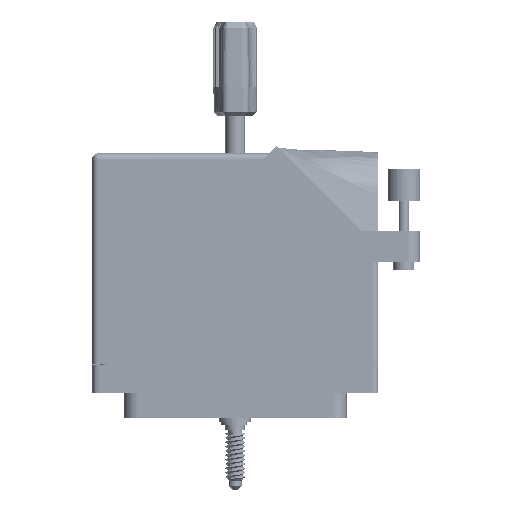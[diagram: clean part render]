
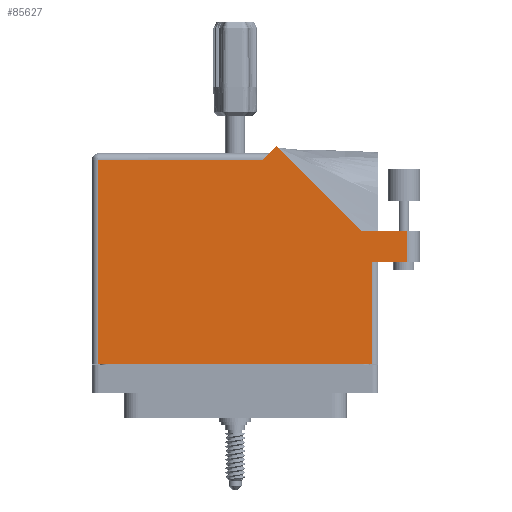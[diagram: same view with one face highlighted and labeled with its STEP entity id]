
A CAD part, front view. The second image highlights one B-rep face of the part: STEP entity #85627.
In plain terms, the highlighted face is planar.
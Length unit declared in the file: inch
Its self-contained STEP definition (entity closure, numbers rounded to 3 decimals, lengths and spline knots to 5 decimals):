
#1533 = VERTEX_POINT ( 'NONE', #86568 ) ;
#3711 = VERTEX_POINT ( 'NONE', #14160 ) ;
#5262 = DIRECTION ( 'NONE',  ( 1., 0., 0. ) ) ;
#7871 = VECTOR ( 'NONE', #48670, 39.37008 ) ;
#8618 = VECTOR ( 'NONE', #37845, 39.37008 ) ;
#8936 = DIRECTION ( 'NONE',  ( -1., 0., 0. ) ) ;
#9308 = CARTESIAN_POINT ( 'NONE',  ( 1.7775, 1.187, 0.765 ) ) ;
#9536 = CARTESIAN_POINT ( 'NONE',  ( 1.6525, 0.88, 0.765 ) ) ;
#9553 = LINE ( 'NONE', #60738, #47862 ) ;
#10353 = ORIENTED_EDGE ( 'NONE', *, *, #39076, .T. ) ;
#11159 = DIRECTION ( 'NONE',  ( 0., 1., 0. ) ) ;
#12064 = VERTEX_POINT ( 'NONE', #9536 ) ;
#12413 = VERTEX_POINT ( 'NONE', #81875 ) ;
#12888 = ORIENTED_EDGE ( 'NONE', *, *, #55813, .T. ) ;
#14160 = CARTESIAN_POINT ( 'NONE',  ( 0.39821, 2.00071, 0.765 ) ) ;
#15164 = VERTEX_POINT ( 'NONE', #15915 ) ;
#15915 = CARTESIAN_POINT ( 'NONE',  ( 1.21192, 1.187, 0.765 ) ) ;
#18569 = EDGE_CURVE ( 'NONE', #64578, #12064, #103659, .T. ) ;
#19129 = CARTESIAN_POINT ( 'NONE',  ( 1.21192, 1.187, 0.765 ) ) ;
#21753 = CARTESIAN_POINT ( 'NONE',  ( -1.3155, -0.1, 0.765 ) ) ;
#22735 = LINE ( 'NONE', #62790, #8618 ) ;
#22827 = VERTEX_POINT ( 'NONE', #45291 ) ;
#23236 = ORIENTED_EDGE ( 'NONE', *, *, #60912, .T. ) ;
#25490 = DIRECTION ( 'NONE',  ( -0.707, -0.707, 0. ) ) ;
#25678 = LINE ( 'NONE', #64691, #7871 ) ;
#25749 = ORIENTED_EDGE ( 'NONE', *, *, #65147, .T. ) ;
#27360 = CARTESIAN_POINT ( 'NONE',  ( -1.3155, 1.868, 0.765 ) ) ;
#29050 = VERTEX_POINT ( 'NONE', #27360 ) ;
#29961 = DIRECTION ( 'NONE',  ( 0., -1., 0. ) ) ;
#31330 = LINE ( 'NONE', #98326, #93917 ) ;
#32808 = ORIENTED_EDGE ( 'NONE', *, *, #70916, .T. ) ;
#34375 = VECTOR ( 'NONE', #29961, 39.37008 ) ;
#34515 = EDGE_CURVE ( 'NONE', #12064, #12413, #25678, .T. ) ;
#35203 = DIRECTION ( 'NONE',  ( -0.707, 0.707, 0. ) ) ;
#37845 = DIRECTION ( 'NONE',  ( -1., 0., 0. ) ) ;
#39076 = EDGE_CURVE ( 'NONE', #3711, #1533, #31330, .T. ) ;
#42021 = CARTESIAN_POINT ( 'NONE',  ( -1.3775, 1.93, 0.765 ) ) ;
#42851 = DIRECTION ( 'NONE',  ( 0., 0., -1. ) ) ;
#45291 = CARTESIAN_POINT ( 'NONE',  ( -1.3155, -0.1, 0.765 ) ) ;
#47862 = VECTOR ( 'NONE', #11159, 39.37008 ) ;
#48670 = DIRECTION ( 'NONE',  ( 0., 1., 0. ) ) ;
#49932 = VECTOR ( 'NONE', #5262, 39.37008 ) ;
#50260 = CARTESIAN_POINT ( 'NONE',  ( 1.3775, 0.88, 0.765 ) ) ;
#51410 = AXIS2_PLACEMENT_3D ( 'NONE', #42021, #42851, #99990 ) ;
#52316 = VERTEX_POINT ( 'NONE', #105827 ) ;
#53189 = LINE ( 'NONE', #19129, #94052 ) ;
#55813 = EDGE_CURVE ( 'NONE', #15164, #3711, #53189, .T. ) ;
#57748 = ORIENTED_EDGE ( 'NONE', *, *, #34515, .T. ) ;
#60051 = ORIENTED_EDGE ( 'NONE', *, *, #105525, .T. ) ;
#60738 = CARTESIAN_POINT ( 'NONE',  ( 1.3155, 0.88, 0.765 ) ) ;
#60912 = EDGE_CURVE ( 'NONE', #29050, #22827, #82968, .T. ) ;
#62097 = VECTOR ( 'NONE', #8936, 39.37008 ) ;
#62790 = CARTESIAN_POINT ( 'NONE',  ( -1.3775, 1.868, 0.765 ) ) ;
#63529 = CARTESIAN_POINT ( 'NONE',  ( 1.3155, 0.88, 0.765 ) ) ;
#63993 = ORIENTED_EDGE ( 'NONE', *, *, #18569, .T. ) ;
#64578 = VERTEX_POINT ( 'NONE', #63529 ) ;
#64691 = CARTESIAN_POINT ( 'NONE',  ( 1.6525, 1.187, 0.765 ) ) ;
#65147 = EDGE_CURVE ( 'NONE', #22827, #52316, #71584, .T. ) ;
#70916 = EDGE_CURVE ( 'NONE', #52316, #64578, #9553, .T. ) ;
#71584 = LINE ( 'NONE', #102746, #49932 ) ;
#79349 = FACE_OUTER_BOUND ( 'NONE', #92042, .T. ) ;
#81875 = CARTESIAN_POINT ( 'NONE',  ( 1.6525, 1.187, 0.765 ) ) ;
#82968 = LINE ( 'NONE', #21753, #34375 ) ;
#85627 = ADVANCED_FACE ( 'NONE', ( #79349 ), #91626, .F. ) ;
#86470 = ORIENTED_EDGE ( 'NONE', *, *, #104288, .T. ) ;
#86568 = CARTESIAN_POINT ( 'NONE',  ( 0.2655, 1.868, 0.765 ) ) ;
#90214 = DIRECTION ( 'NONE',  ( 1., 0., 0. ) ) ;
#91626 = PLANE ( 'NONE',  #51410 ) ;
#92042 = EDGE_LOOP ( 'NONE', ( #63993, #57748, #60051, #12888, #10353, #86470, #23236, #25749, #32808 ) ) ;
#93917 = VECTOR ( 'NONE', #25490, 39.37008 ) ;
#94052 = VECTOR ( 'NONE', #35203, 39.37008 ) ;
#98326 = CARTESIAN_POINT ( 'NONE',  ( 0.3275, 1.93, 0.765 ) ) ;
#99990 = DIRECTION ( 'NONE',  ( -1., 0., 0. ) ) ;
#101100 = VECTOR ( 'NONE', #90214, 39.37008 ) ;
#102746 = CARTESIAN_POINT ( 'NONE',  ( -1.3775, -0.1, 0.765 ) ) ;
#103659 = LINE ( 'NONE', #50260, #101100 ) ;
#104288 = EDGE_CURVE ( 'NONE', #1533, #29050, #22735, .T. ) ;
#105525 = EDGE_CURVE ( 'NONE', #12413, #15164, #105565, .T. ) ;
#105565 = LINE ( 'NONE', #9308, #62097 ) ;
#105827 = CARTESIAN_POINT ( 'NONE',  ( 1.3155, -0.1, 0.765 ) ) ;
